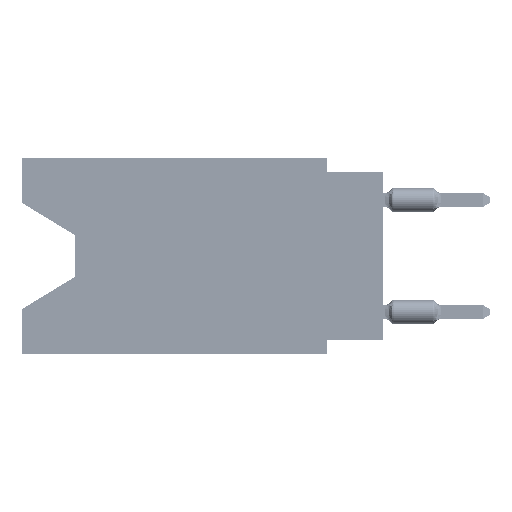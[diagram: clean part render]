
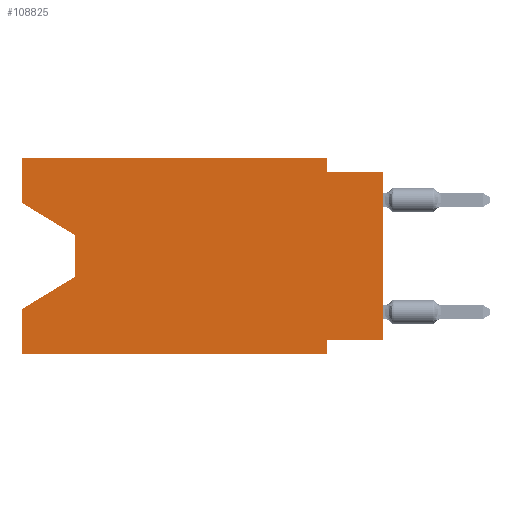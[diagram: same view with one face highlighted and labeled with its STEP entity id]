
A CAD part, left-side view. The second image highlights one B-rep face of the part: STEP entity #108825.
In plain terms, the highlighted planar face has unit normal (-1, 0, 0).
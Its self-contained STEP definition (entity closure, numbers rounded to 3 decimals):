
#106 = ORIENTED_EDGE ( 'NONE', *, *, #18424, .T. ) ;
#2070 = CARTESIAN_POINT ( 'NONE',  ( 0., 16.383, -6.852 ) ) ;
#2164 = ORIENTED_EDGE ( 'NONE', *, *, #84102, .F. ) ;
#2598 = ORIENTED_EDGE ( 'NONE', *, *, #12367, .T. ) ;
#3474 = CARTESIAN_POINT ( 'NONE',  ( 0., 16.383, -8.89 ) ) ;
#4264 = CARTESIAN_POINT ( 'NONE',  ( 0., 13.97, -5.385 ) ) ;
#4485 = VERTEX_POINT ( 'NONE', #60890 ) ;
#9989 = DIRECTION ( 'NONE',  ( 0., 0., -1. ) ) ;
#11116 = CARTESIAN_POINT ( 'NONE',  ( 0., 13.97, -3.505 ) ) ;
#11752 = CARTESIAN_POINT ( 'NONE',  ( 0., 2.54, 0. ) ) ;
#12301 = DIRECTION ( 'NONE',  ( 0., -1., 0. ) ) ;
#12367 = EDGE_CURVE ( 'NONE', #4485, #25481, #69895, .T. ) ;
#14600 = CARTESIAN_POINT ( 'NONE',  ( 0., 16.383, 0. ) ) ;
#14686 = EDGE_CURVE ( 'NONE', #24638, #107935, #89398, .T. ) ;
#17013 = CARTESIAN_POINT ( 'NONE',  ( 0., 2.54, -8.89 ) ) ;
#17629 = VECTOR ( 'NONE', #9989, 1000. ) ;
#18424 = EDGE_CURVE ( 'NONE', #61947, #81165, #98424, .T. ) ;
#19696 = EDGE_CURVE ( 'NONE', #49665, #54484, #51662, .T. ) ;
#21247 = LINE ( 'NONE', #30613, #109927 ) ;
#22314 = DIRECTION ( 'NONE',  ( 0., 0., 1. ) ) ;
#23123 = EDGE_LOOP ( 'NONE', ( #2598, #100663, #95722, #25772, #106, #51267, #79236, #74401, #58558, #2164, #77917, #72269 ) ) ;
#24638 = VERTEX_POINT ( 'NONE', #58253 ) ;
#24781 = VECTOR ( 'NONE', #110175, 1000. ) ;
#25481 = VERTEX_POINT ( 'NONE', #11116 ) ;
#25772 = ORIENTED_EDGE ( 'NONE', *, *, #77641, .F. ) ;
#27150 = CARTESIAN_POINT ( 'NONE',  ( 0., 0., -8.255 ) ) ;
#27904 = VERTEX_POINT ( 'NONE', #103544 ) ;
#28999 = VECTOR ( 'NONE', #12301, 1000. ) ;
#30613 = CARTESIAN_POINT ( 'NONE',  ( 0., 16.383, 0. ) ) ;
#34465 = CARTESIAN_POINT ( 'NONE',  ( 0., 16.383, -8.89 ) ) ;
#36958 = VECTOR ( 'NONE', #106147, 1000. ) ;
#38517 = VECTOR ( 'NONE', #52678, 1000. ) ;
#42109 = CARTESIAN_POINT ( 'NONE',  ( 0., 13.97, -5.385 ) ) ;
#46129 = LINE ( 'NONE', #11752, #17629 ) ;
#46563 = CARTESIAN_POINT ( 'NONE',  ( 0., 2.54, -8.255 ) ) ;
#47943 = LINE ( 'NONE', #66895, #24781 ) ;
#49025 = CARTESIAN_POINT ( 'NONE',  ( 0., 0., -0.635 ) ) ;
#49665 = VERTEX_POINT ( 'NONE', #42109 ) ;
#50118 = CARTESIAN_POINT ( 'NONE',  ( 0., 0., 0. ) ) ;
#50430 = CARTESIAN_POINT ( 'NONE',  ( 0., 2.54, -8.89 ) ) ;
#51267 = ORIENTED_EDGE ( 'NONE', *, *, #110920, .F. ) ;
#51539 = DIRECTION ( 'NONE',  ( 0., -0.855, -0.519 ) ) ;
#51662 = LINE ( 'NONE', #4264, #56088 ) ;
#52678 = DIRECTION ( 'NONE',  ( 0., 1., 0. ) ) ;
#52834 = EDGE_CURVE ( 'NONE', #97640, #64403, #21247, .T. ) ;
#53160 = DIRECTION ( 'NONE',  ( 0., 0., -1. ) ) ;
#54484 = VERTEX_POINT ( 'NONE', #2070 ) ;
#56088 = VECTOR ( 'NONE', #68847, 1000. ) ;
#56474 = AXIS2_PLACEMENT_3D ( 'NONE', #91898, #73552, #57538 ) ;
#57538 = DIRECTION ( 'NONE',  ( 0., 0., -1. ) ) ;
#58253 = CARTESIAN_POINT ( 'NONE',  ( 0., 0., -8.255 ) ) ;
#58432 = DIRECTION ( 'NONE',  ( 0., 0., 1. ) ) ;
#58558 = ORIENTED_EDGE ( 'NONE', *, *, #104642, .F. ) ;
#59041 = DIRECTION ( 'NONE',  ( 0., -1., 0. ) ) ;
#60011 = EDGE_CURVE ( 'NONE', #24638, #27904, #85091, .T. ) ;
#60890 = CARTESIAN_POINT ( 'NONE',  ( 0., 16.383, -2.038 ) ) ;
#61814 = CARTESIAN_POINT ( 'NONE',  ( 0., 13.97, -3.505 ) ) ;
#61947 = VERTEX_POINT ( 'NONE', #3474 ) ;
#62054 = LINE ( 'NONE', #17013, #104164 ) ;
#64403 = VERTEX_POINT ( 'NONE', #94450 ) ;
#66422 = PLANE ( 'NONE',  #56474 ) ;
#66895 = CARTESIAN_POINT ( 'NONE',  ( 0., 16.383, 0. ) ) ;
#68847 = DIRECTION ( 'NONE',  ( 0., 0.855, -0.519 ) ) ;
#69895 = LINE ( 'NONE', #71058, #100504 ) ;
#71058 = CARTESIAN_POINT ( 'NONE',  ( 0., 16.383, -2.038 ) ) ;
#71925 = CARTESIAN_POINT ( 'NONE',  ( 0., 2.54, -0.635 ) ) ;
#72269 = ORIENTED_EDGE ( 'NONE', *, *, #101926, .F. ) ;
#72440 = DIRECTION ( 'NONE',  ( 0., 0., -1. ) ) ;
#73552 = DIRECTION ( 'NONE',  ( 1., 0., 0. ) ) ;
#74401 = ORIENTED_EDGE ( 'NONE', *, *, #60011, .T. ) ;
#77451 = LINE ( 'NONE', #49025, #28999 ) ;
#77641 = EDGE_CURVE ( 'NONE', #61947, #54484, #104080, .T. ) ;
#77917 = ORIENTED_EDGE ( 'NONE', *, *, #52834, .F. ) ;
#79236 = ORIENTED_EDGE ( 'NONE', *, *, #14686, .F. ) ;
#80754 = VECTOR ( 'NONE', #58432, 1000. ) ;
#81165 = VERTEX_POINT ( 'NONE', #50430 ) ;
#81890 = LINE ( 'NONE', #61814, #113092 ) ;
#84102 = EDGE_CURVE ( 'NONE', #64403, #91459, #46129, .T. ) ;
#85091 = LINE ( 'NONE', #50118, #80754 ) ;
#89398 = LINE ( 'NONE', #27150, #38517 ) ;
#91459 = VERTEX_POINT ( 'NONE', #71925 ) ;
#91898 = CARTESIAN_POINT ( 'NONE',  ( 0., 16.383, 0. ) ) ;
#94450 = CARTESIAN_POINT ( 'NONE',  ( 0., 2.54, 0. ) ) ;
#95722 = ORIENTED_EDGE ( 'NONE', *, *, #19696, .T. ) ;
#96633 = EDGE_CURVE ( 'NONE', #25481, #49665, #81890, .T. ) ;
#97640 = VERTEX_POINT ( 'NONE', #111217 ) ;
#98424 = LINE ( 'NONE', #34465, #36958 ) ;
#99948 = VECTOR ( 'NONE', #22314, 1000. ) ;
#100504 = VECTOR ( 'NONE', #51539, 1000. ) ;
#100663 = ORIENTED_EDGE ( 'NONE', *, *, #96633, .T. ) ;
#101926 = EDGE_CURVE ( 'NONE', #4485, #97640, #47943, .T. ) ;
#103544 = CARTESIAN_POINT ( 'NONE',  ( 0., 0., -0.635 ) ) ;
#104080 = LINE ( 'NONE', #14600, #99948 ) ;
#104164 = VECTOR ( 'NONE', #53160, 1000. ) ;
#104642 = EDGE_CURVE ( 'NONE', #91459, #27904, #77451, .T. ) ;
#106147 = DIRECTION ( 'NONE',  ( 0., -1., 0. ) ) ;
#107935 = VERTEX_POINT ( 'NONE', #46563 ) ;
#108825 = ADVANCED_FACE ( 'NONE', ( #111437 ), #66422, .F. ) ;
#109927 = VECTOR ( 'NONE', #59041, 1000. ) ;
#110175 = DIRECTION ( 'NONE',  ( 0., 0., 1. ) ) ;
#110920 = EDGE_CURVE ( 'NONE', #107935, #81165, #62054, .T. ) ;
#111217 = CARTESIAN_POINT ( 'NONE',  ( 0., 16.383, 0. ) ) ;
#111437 = FACE_OUTER_BOUND ( 'NONE', #23123, .T. ) ;
#113092 = VECTOR ( 'NONE', #72440, 1000. ) ;
